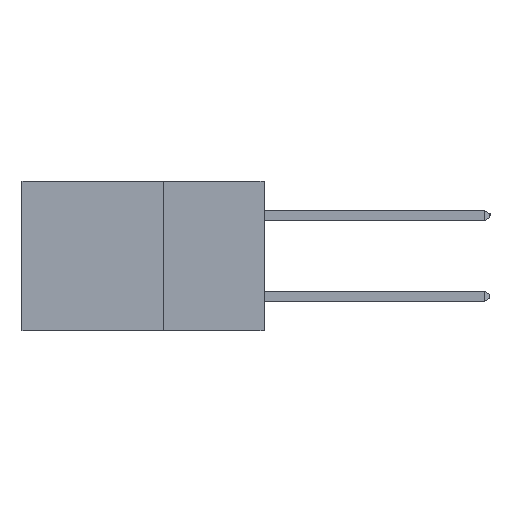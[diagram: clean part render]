
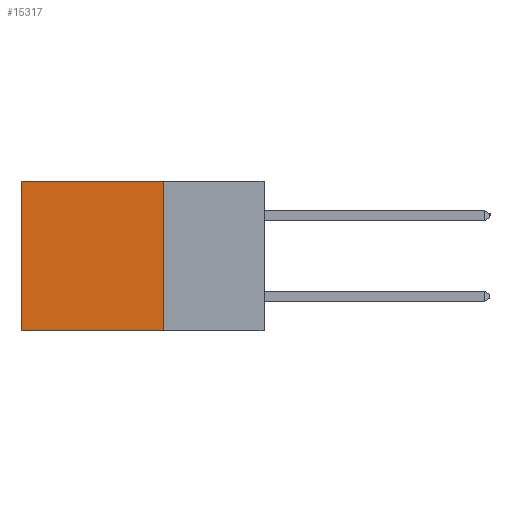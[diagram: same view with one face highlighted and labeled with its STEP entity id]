
A CAD part, left-side view. The second image highlights one B-rep face of the part: STEP entity #15317.
In plain terms, the highlighted planar face has unit normal (-1, 0, 0).
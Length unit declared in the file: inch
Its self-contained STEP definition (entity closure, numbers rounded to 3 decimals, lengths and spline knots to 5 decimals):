
#459 = ORIENTED_EDGE ( 'NONE', *, *, #14401, .F. ) ;
#821 = DIRECTION ( 'NONE',  ( 0., 0., -1. ) ) ;
#1157 = EDGE_LOOP ( 'NONE', ( #16105, #19643, #459, #5691 ) ) ;
#1913 = EDGE_CURVE ( 'NONE', #17658, #18497, #18004, .T. ) ;
#3286 = VECTOR ( 'NONE', #14511, 39.37008 ) ;
#3867 = PLANE ( 'NONE',  #19950 ) ;
#5116 = DIRECTION ( 'NONE',  ( 1., 0., 0. ) ) ;
#5472 = CARTESIAN_POINT ( 'NONE',  ( 0.2615, 0.25, -0.37 ) ) ;
#5686 = VECTOR ( 'NONE', #13440, 39.37008 ) ;
#5691 = ORIENTED_EDGE ( 'NONE', *, *, #9420, .T. ) ;
#7643 = CARTESIAN_POINT ( 'NONE',  ( 0.2615, 0.25, -0.37 ) ) ;
#8669 = LINE ( 'NONE', #20668, #5686 ) ;
#9420 = EDGE_CURVE ( 'NONE', #19410, #17658, #8669, .T. ) ;
#9750 = LINE ( 'NONE', #16681, #17346 ) ;
#10872 = CARTESIAN_POINT ( 'NONE',  ( 0.2615, 0.6, -0.37 ) ) ;
#11077 = LINE ( 'NONE', #14508, #13820 ) ;
#13440 = DIRECTION ( 'NONE',  ( 0., 1., 0. ) ) ;
#13820 = VECTOR ( 'NONE', #821, 39.37008 ) ;
#13875 = DIRECTION ( 'NONE',  ( 0., 0., -1. ) ) ;
#14401 = EDGE_CURVE ( 'NONE', #19410, #15712, #11077, .T. ) ;
#14508 = CARTESIAN_POINT ( 'NONE',  ( 0.2615, 0.25, -0.37 ) ) ;
#14511 = DIRECTION ( 'NONE',  ( 0., 0., -1. ) ) ;
#15317 = ADVANCED_FACE ( 'NONE', ( #21016 ), #3867, .F. ) ;
#15379 = CARTESIAN_POINT ( 'NONE',  ( 0.2615, 0.25, 0. ) ) ;
#15394 = DIRECTION ( 'NONE',  ( 0., 1., 0. ) ) ;
#15712 = VERTEX_POINT ( 'NONE', #7643 ) ;
#16105 = ORIENTED_EDGE ( 'NONE', *, *, #1913, .T. ) ;
#16681 = CARTESIAN_POINT ( 'NONE',  ( 0.2615, 0.25, -0.37 ) ) ;
#17346 = VECTOR ( 'NONE', #15394, 39.37008 ) ;
#17658 = VERTEX_POINT ( 'NONE', #21883 ) ;
#18004 = LINE ( 'NONE', #10872, #3286 ) ;
#18497 = VERTEX_POINT ( 'NONE', #20431 ) ;
#19410 = VERTEX_POINT ( 'NONE', #15379 ) ;
#19643 = ORIENTED_EDGE ( 'NONE', *, *, #21935, .F. ) ;
#19950 = AXIS2_PLACEMENT_3D ( 'NONE', #5472, #5116, #13875 ) ;
#20431 = CARTESIAN_POINT ( 'NONE',  ( 0.2615, 0.6, -0.37 ) ) ;
#20668 = CARTESIAN_POINT ( 'NONE',  ( 0.2615, 0.25, 0. ) ) ;
#21016 = FACE_OUTER_BOUND ( 'NONE', #1157, .T. ) ;
#21883 = CARTESIAN_POINT ( 'NONE',  ( 0.2615, 0.6, 0. ) ) ;
#21935 = EDGE_CURVE ( 'NONE', #15712, #18497, #9750, .T. ) ;
